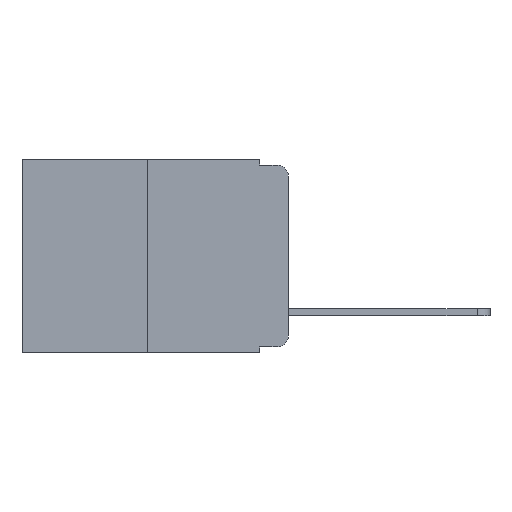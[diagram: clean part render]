
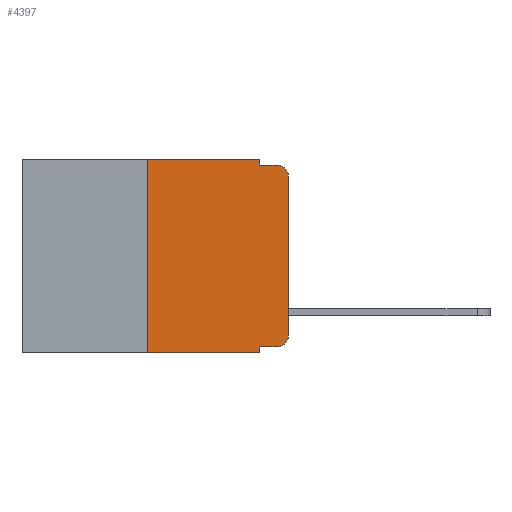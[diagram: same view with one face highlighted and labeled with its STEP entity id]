
A CAD part, left-side view. The second image highlights one B-rep face of the part: STEP entity #4397.
In plain terms, the highlighted planar face has unit normal (-1, 0, 0).
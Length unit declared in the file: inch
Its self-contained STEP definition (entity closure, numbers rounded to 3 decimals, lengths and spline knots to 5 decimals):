
#2 = ORIENTED_EDGE ( 'NONE', *, *, #10084, .T. ) ;
#70 = CARTESIAN_POINT ( 'NONE',  ( 0., 0.051, 0. ) ) ;
#153 = VERTEX_POINT ( 'NONE', #779 ) ;
#256 = VERTEX_POINT ( 'NONE', #2405 ) ;
#356 = DIRECTION ( 'NONE',  ( 0., 0., -1. ) ) ;
#361 = CARTESIAN_POINT ( 'NONE',  ( 0., 0.051, -0.343 ) ) ;
#422 = VERTEX_POINT ( 'NONE', #3906 ) ;
#467 = LINE ( 'NONE', #1138, #8647 ) ;
#625 = DIRECTION ( 'NONE',  ( 0., -1., 0. ) ) ;
#737 = ORIENTED_EDGE ( 'NONE', *, *, #9830, .T. ) ;
#745 = ORIENTED_EDGE ( 'NONE', *, *, #4278, .F. ) ;
#767 = CARTESIAN_POINT ( 'NONE',  ( 0., 0.25, 0. ) ) ;
#779 = CARTESIAN_POINT ( 'NONE',  ( 0., 0.25, -0.343 ) ) ;
#868 = DIRECTION ( 'NONE',  ( 0., 0., 1. ) ) ;
#873 = ORIENTED_EDGE ( 'NONE', *, *, #4802, .F. ) ;
#1066 = EDGE_CURVE ( 'NONE', #1192, #5945, #467, .T. ) ;
#1138 = CARTESIAN_POINT ( 'NONE',  ( 0., 0.051, -0.01 ) ) ;
#1139 = ORIENTED_EDGE ( 'NONE', *, *, #6305, .T. ) ;
#1192 = VERTEX_POINT ( 'NONE', #2477 ) ;
#1216 = FACE_OUTER_BOUND ( 'NONE', #8249, .T. ) ;
#1314 = CIRCLE ( 'NONE', #7544, 0.02 ) ;
#1438 = EDGE_CURVE ( 'NONE', #4533, #1192, #4295, .T. ) ;
#1630 = EDGE_CURVE ( 'NONE', #3309, #4533, #6509, .T. ) ;
#1664 = CARTESIAN_POINT ( 'NONE',  ( 0., 0., 0. ) ) ;
#1730 = LINE ( 'NONE', #9680, #9676 ) ;
#1743 = CARTESIAN_POINT ( 'NONE',  ( 0., 0.473, 0. ) ) ;
#2068 = EDGE_CURVE ( 'NONE', #3879, #256, #7402, .T. ) ;
#2161 = AXIS2_PLACEMENT_3D ( 'NONE', #6328, #8695, #7014 ) ;
#2395 = EDGE_CURVE ( 'NONE', #256, #5945, #7053, .T. ) ;
#2405 = CARTESIAN_POINT ( 'NONE',  ( 0., 0., -0.03 ) ) ;
#2464 = DIRECTION ( 'NONE',  ( 0., -1., 0. ) ) ;
#2477 = CARTESIAN_POINT ( 'NONE',  ( 0., 0.051, -0.01 ) ) ;
#2563 = ORIENTED_EDGE ( 'NONE', *, *, #2395, .T. ) ;
#2836 = DIRECTION ( 'NONE',  ( -1., 0., 0. ) ) ;
#2860 = VECTOR ( 'NONE', #625, 39.37008 ) ;
#2945 = ORIENTED_EDGE ( 'NONE', *, *, #1066, .F. ) ;
#3040 = ORIENTED_EDGE ( 'NONE', *, *, #2068, .T. ) ;
#3309 = VERTEX_POINT ( 'NONE', #767 ) ;
#3679 = CARTESIAN_POINT ( 'NONE',  ( 0., 0., -0.313 ) ) ;
#3722 = ORIENTED_EDGE ( 'NONE', *, *, #1438, .F. ) ;
#3879 = VERTEX_POINT ( 'NONE', #3679 ) ;
#3906 = CARTESIAN_POINT ( 'NONE',  ( 0., 0.051, -0.333 ) ) ;
#3980 = CARTESIAN_POINT ( 'NONE',  ( 0., 0.473, -0.343 ) ) ;
#4075 = VERTEX_POINT ( 'NONE', #361 ) ;
#4278 = EDGE_CURVE ( 'NONE', #422, #4075, #5249, .T. ) ;
#4295 = LINE ( 'NONE', #70, #7858 ) ;
#4397 = ADVANCED_FACE ( 'NONE', ( #1216 ), #8330, .F. ) ;
#4428 = VECTOR ( 'NONE', #5248, 39.37008 ) ;
#4533 = VERTEX_POINT ( 'NONE', #5059 ) ;
#4651 = VECTOR ( 'NONE', #6844, 39.37008 ) ;
#4666 = ORIENTED_EDGE ( 'NONE', *, *, #1630, .F. ) ;
#4802 = EDGE_CURVE ( 'NONE', #153, #3309, #1730, .T. ) ;
#4876 = CARTESIAN_POINT ( 'NONE',  ( 0., 0.02, -0.333 ) ) ;
#5024 = CARTESIAN_POINT ( 'NONE',  ( 0., 0.02, -0.01 ) ) ;
#5059 = CARTESIAN_POINT ( 'NONE',  ( 0., 0.051, 0. ) ) ;
#5082 = LINE ( 'NONE', #3980, #2860 ) ;
#5143 = AXIS2_PLACEMENT_3D ( 'NONE', #7956, #8358, #8067 ) ;
#5177 = VECTOR ( 'NONE', #868, 39.37008 ) ;
#5248 = DIRECTION ( 'NONE',  ( 0., -1., 0. ) ) ;
#5249 = LINE ( 'NONE', #6505, #6787 ) ;
#5945 = VERTEX_POINT ( 'NONE', #5024 ) ;
#6305 = EDGE_CURVE ( 'NONE', #422, #7373, #6701, .T. ) ;
#6328 = CARTESIAN_POINT ( 'NONE',  ( 0., 0.473, 0. ) ) ;
#6505 = CARTESIAN_POINT ( 'NONE',  ( 0., 0.051, 0. ) ) ;
#6509 = LINE ( 'NONE', #1743, #4428 ) ;
#6701 = LINE ( 'NONE', #10066, #4651 ) ;
#6787 = VECTOR ( 'NONE', #356, 39.37008 ) ;
#6844 = DIRECTION ( 'NONE',  ( 0., -1., 0. ) ) ;
#7014 = DIRECTION ( 'NONE',  ( 0., 0., -1. ) ) ;
#7053 = CIRCLE ( 'NONE', #5143, 0.02 ) ;
#7369 = DIRECTION ( 'NONE',  ( 0., 0., -1. ) ) ;
#7373 = VERTEX_POINT ( 'NONE', #4876 ) ;
#7402 = LINE ( 'NONE', #1664, #5177 ) ;
#7544 = AXIS2_PLACEMENT_3D ( 'NONE', #7549, #2836, #8286 ) ;
#7549 = CARTESIAN_POINT ( 'NONE',  ( 0., 0.02, -0.313 ) ) ;
#7858 = VECTOR ( 'NONE', #7369, 39.37008 ) ;
#7956 = CARTESIAN_POINT ( 'NONE',  ( 0., 0.02, -0.03 ) ) ;
#8067 = DIRECTION ( 'NONE',  ( 0., 0., -1. ) ) ;
#8249 = EDGE_LOOP ( 'NONE', ( #3040, #2563, #2945, #3722, #4666, #873, #2, #745, #1139, #737 ) ) ;
#8286 = DIRECTION ( 'NONE',  ( 0., 0., -1. ) ) ;
#8330 = PLANE ( 'NONE',  #2161 ) ;
#8358 = DIRECTION ( 'NONE',  ( -1., 0., 0. ) ) ;
#8647 = VECTOR ( 'NONE', #2464, 39.37008 ) ;
#8648 = DIRECTION ( 'NONE',  ( 0., 0., 1. ) ) ;
#8695 = DIRECTION ( 'NONE',  ( 1., 0., 0. ) ) ;
#9676 = VECTOR ( 'NONE', #8648, 39.37008 ) ;
#9680 = CARTESIAN_POINT ( 'NONE',  ( 0., 0.25, 0. ) ) ;
#9830 = EDGE_CURVE ( 'NONE', #7373, #3879, #1314, .T. ) ;
#10066 = CARTESIAN_POINT ( 'NONE',  ( 0., 0.051, -0.333 ) ) ;
#10084 = EDGE_CURVE ( 'NONE', #153, #4075, #5082, .T. ) ;
